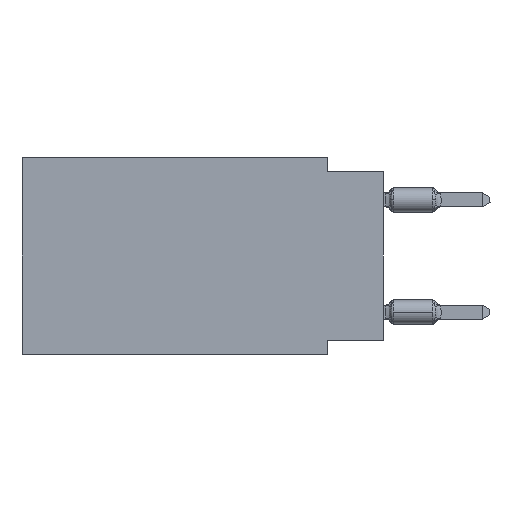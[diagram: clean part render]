
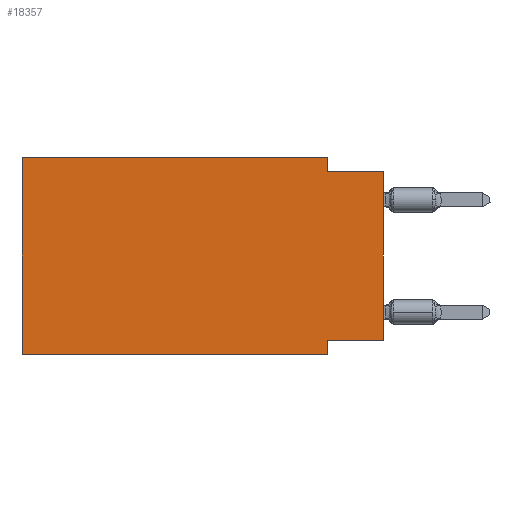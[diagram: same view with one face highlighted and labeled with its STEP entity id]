
A CAD part, left-side view. The second image highlights one B-rep face of the part: STEP entity #18357.
In plain terms, the highlighted planar face has unit normal (-1, 0, 0).
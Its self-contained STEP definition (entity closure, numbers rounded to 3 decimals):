
#238 = EDGE_CURVE ( 'NONE', #1345, #2116, #16691, .T. ) ;
#472 = LINE ( 'NONE', #5321, #8289 ) ;
#1304 = ORIENTED_EDGE ( 'NONE', *, *, #238, .T. ) ;
#1332 = CARTESIAN_POINT ( 'NONE',  ( 0., 16.383, 0. ) ) ;
#1345 = VERTEX_POINT ( 'NONE', #11541 ) ;
#2116 = VERTEX_POINT ( 'NONE', #4181 ) ;
#2405 = DIRECTION ( 'NONE',  ( 0., 0., -1. ) ) ;
#2417 = EDGE_CURVE ( 'NONE', #5973, #6123, #7162, .T. ) ;
#2435 = CARTESIAN_POINT ( 'NONE',  ( 0., 2.54, -8.255 ) ) ;
#2748 = DIRECTION ( 'NONE',  ( 0., 0., -1. ) ) ;
#2967 = CARTESIAN_POINT ( 'NONE',  ( 0., 0., 0. ) ) ;
#3646 = EDGE_CURVE ( 'NONE', #1345, #9324, #18271, .T. ) ;
#3707 = VECTOR ( 'NONE', #16771, 1000. ) ;
#3746 = CARTESIAN_POINT ( 'NONE',  ( 0., 16.383, -8.89 ) ) ;
#4181 = CARTESIAN_POINT ( 'NONE',  ( 0., 0., -0.635 ) ) ;
#4483 = ORIENTED_EDGE ( 'NONE', *, *, #17845, .F. ) ;
#4733 = ORIENTED_EDGE ( 'NONE', *, *, #9309, .T. ) ;
#4930 = ORIENTED_EDGE ( 'NONE', *, *, #14055, .F. ) ;
#5321 = CARTESIAN_POINT ( 'NONE',  ( 0., 16.383, 0. ) ) ;
#5496 = ORIENTED_EDGE ( 'NONE', *, *, #2417, .F. ) ;
#5812 = ORIENTED_EDGE ( 'NONE', *, *, #3646, .F. ) ;
#5973 = VERTEX_POINT ( 'NONE', #3746 ) ;
#6123 = VERTEX_POINT ( 'NONE', #1332 ) ;
#6631 = DIRECTION ( 'NONE',  ( 0., -1., 0. ) ) ;
#6880 = EDGE_CURVE ( 'NONE', #6123, #13171, #472, .T. ) ;
#6971 = DIRECTION ( 'NONE',  ( 0., -1., 0. ) ) ;
#7162 = LINE ( 'NONE', #10591, #16331 ) ;
#7202 = DIRECTION ( 'NONE',  ( 0., -1., 0. ) ) ;
#7327 = VECTOR ( 'NONE', #19710, 1000. ) ;
#7387 = LINE ( 'NONE', #10309, #14458 ) ;
#7517 = ORIENTED_EDGE ( 'NONE', *, *, #12934, .F. ) ;
#8168 = CARTESIAN_POINT ( 'NONE',  ( 0., 2.54, 0. ) ) ;
#8289 = VECTOR ( 'NONE', #6631, 1000. ) ;
#8576 = LINE ( 'NONE', #9991, #14914 ) ;
#8765 = CARTESIAN_POINT ( 'NONE',  ( 0., 16.383, 0. ) ) ;
#9309 = EDGE_CURVE ( 'NONE', #5973, #13697, #13547, .T. ) ;
#9324 = VERTEX_POINT ( 'NONE', #2435 ) ;
#9991 = CARTESIAN_POINT ( 'NONE',  ( 0., 2.54, 0. ) ) ;
#10309 = CARTESIAN_POINT ( 'NONE',  ( 0., 2.54, -8.89 ) ) ;
#10366 = CARTESIAN_POINT ( 'NONE',  ( 0., 2.54, -8.89 ) ) ;
#10591 = CARTESIAN_POINT ( 'NONE',  ( 0., 16.383, 0. ) ) ;
#11366 = DIRECTION ( 'NONE',  ( 0., 0., -1. ) ) ;
#11541 = CARTESIAN_POINT ( 'NONE',  ( 0., 0., -8.255 ) ) ;
#12030 = CARTESIAN_POINT ( 'NONE',  ( 0., 16.383, -8.89 ) ) ;
#12124 = CARTESIAN_POINT ( 'NONE',  ( 0., 0., -8.255 ) ) ;
#12934 = EDGE_CURVE ( 'NONE', #9324, #13697, #7387, .T. ) ;
#13171 = VERTEX_POINT ( 'NONE', #8168 ) ;
#13516 = VECTOR ( 'NONE', #6971, 1000. ) ;
#13547 = LINE ( 'NONE', #12030, #13516 ) ;
#13697 = VERTEX_POINT ( 'NONE', #10366 ) ;
#14055 = EDGE_CURVE ( 'NONE', #16169, #2116, #14673, .T. ) ;
#14407 = EDGE_LOOP ( 'NONE', ( #1304, #4930, #4483, #15222, #5496, #4733, #7517, #5812 ) ) ;
#14458 = VECTOR ( 'NONE', #2748, 1000. ) ;
#14551 = CARTESIAN_POINT ( 'NONE',  ( 0., 2.54, -0.635 ) ) ;
#14673 = LINE ( 'NONE', #14878, #16096 ) ;
#14804 = FACE_OUTER_BOUND ( 'NONE', #14407, .T. ) ;
#14878 = CARTESIAN_POINT ( 'NONE',  ( 0., 0., -0.635 ) ) ;
#14914 = VECTOR ( 'NONE', #2405, 1000. ) ;
#14930 = DIRECTION ( 'NONE',  ( 0., 0., 1. ) ) ;
#15222 = ORIENTED_EDGE ( 'NONE', *, *, #6880, .F. ) ;
#15562 = AXIS2_PLACEMENT_3D ( 'NONE', #8765, #16203, #11366 ) ;
#16096 = VECTOR ( 'NONE', #7202, 1000. ) ;
#16106 = PLANE ( 'NONE',  #15562 ) ;
#16169 = VERTEX_POINT ( 'NONE', #14551 ) ;
#16203 = DIRECTION ( 'NONE',  ( 1., 0., 0. ) ) ;
#16331 = VECTOR ( 'NONE', #14930, 1000. ) ;
#16691 = LINE ( 'NONE', #2967, #7327 ) ;
#16771 = DIRECTION ( 'NONE',  ( 0., 1., 0. ) ) ;
#17845 = EDGE_CURVE ( 'NONE', #13171, #16169, #8576, .T. ) ;
#18271 = LINE ( 'NONE', #12124, #3707 ) ;
#18357 = ADVANCED_FACE ( 'NONE', ( #14804 ), #16106, .F. ) ;
#19710 = DIRECTION ( 'NONE',  ( 0., 0., 1. ) ) ;
